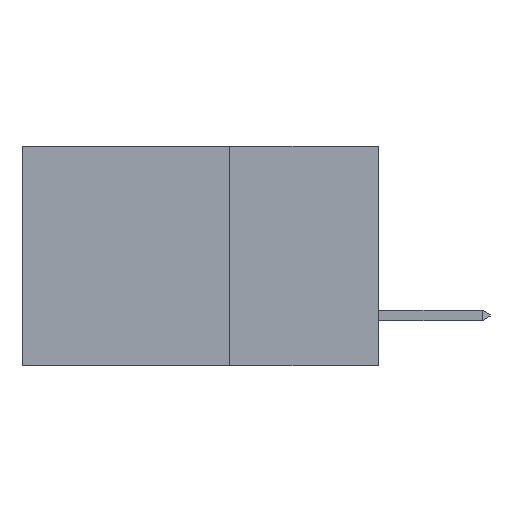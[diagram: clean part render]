
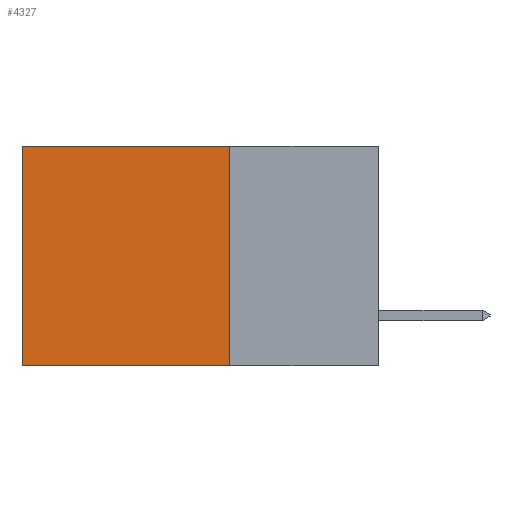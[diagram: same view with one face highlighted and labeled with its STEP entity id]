
A CAD part, left-side view. The second image highlights one B-rep face of the part: STEP entity #4327.
In plain terms, the highlighted planar face has unit normal (-1, 0, 0).
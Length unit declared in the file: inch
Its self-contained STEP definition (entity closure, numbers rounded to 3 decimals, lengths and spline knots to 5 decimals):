
#292 = CARTESIAN_POINT ( 'NONE',  ( 0.298, 0.6, 0. ) ) ;
#398 = ORIENTED_EDGE ( 'NONE', *, *, #7558, .F. ) ;
#803 = CARTESIAN_POINT ( 'NONE',  ( 0.298, 0.25, -0.37 ) ) ;
#1731 = VERTEX_POINT ( 'NONE', #292 ) ;
#1774 = LINE ( 'NONE', #9603, #13063 ) ;
#1909 = PLANE ( 'NONE',  #6850 ) ;
#1918 = DIRECTION ( 'NONE',  ( 0., 1., 0. ) ) ;
#2170 = LINE ( 'NONE', #9643, #13429 ) ;
#2291 = EDGE_CURVE ( 'NONE', #11576, #1731, #2170, .T. ) ;
#2690 = VERTEX_POINT ( 'NONE', #10910 ) ;
#2982 = CARTESIAN_POINT ( 'NONE',  ( 0.298, 0.25, 0. ) ) ;
#4133 = DIRECTION ( 'NONE',  ( 0., 0., -1. ) ) ;
#4327 = ADVANCED_FACE ( 'NONE', ( #7727 ), #1909, .F. ) ;
#5617 = VECTOR ( 'NONE', #13865, 39.37008 ) ;
#6338 = CARTESIAN_POINT ( 'NONE',  ( 0.298, 0.25, 0. ) ) ;
#6403 = ORIENTED_EDGE ( 'NONE', *, *, #2291, .T. ) ;
#6850 = AXIS2_PLACEMENT_3D ( 'NONE', #12520, #6903, #7182 ) ;
#6903 = DIRECTION ( 'NONE',  ( 1., 0., 0. ) ) ;
#7018 = EDGE_LOOP ( 'NONE', ( #10894, #398, #13542, #6403 ) ) ;
#7182 = DIRECTION ( 'NONE',  ( 0., 0., -1. ) ) ;
#7558 = EDGE_CURVE ( 'NONE', #9398, #2690, #1774, .T. ) ;
#7727 = FACE_OUTER_BOUND ( 'NONE', #7018, .T. ) ;
#9398 = VERTEX_POINT ( 'NONE', #803 ) ;
#9548 = CARTESIAN_POINT ( 'NONE',  ( 0.298, 0.6, 0. ) ) ;
#9603 = CARTESIAN_POINT ( 'NONE',  ( 0.298, 0.25, -0.37 ) ) ;
#9643 = CARTESIAN_POINT ( 'NONE',  ( 0.298, 0.25, 0. ) ) ;
#9719 = DIRECTION ( 'NONE',  ( 0., 1., 0. ) ) ;
#10393 = EDGE_CURVE ( 'NONE', #1731, #2690, #12503, .T. ) ;
#10699 = LINE ( 'NONE', #6338, #5617 ) ;
#10894 = ORIENTED_EDGE ( 'NONE', *, *, #10393, .T. ) ;
#10910 = CARTESIAN_POINT ( 'NONE',  ( 0.298, 0.6, -0.37 ) ) ;
#11576 = VERTEX_POINT ( 'NONE', #2982 ) ;
#11857 = VECTOR ( 'NONE', #4133, 39.37008 ) ;
#12503 = LINE ( 'NONE', #9548, #11857 ) ;
#12520 = CARTESIAN_POINT ( 'NONE',  ( 0.298, 0.25, 0. ) ) ;
#13063 = VECTOR ( 'NONE', #1918, 39.37008 ) ;
#13429 = VECTOR ( 'NONE', #9719, 39.37008 ) ;
#13542 = ORIENTED_EDGE ( 'NONE', *, *, #13974, .F. ) ;
#13865 = DIRECTION ( 'NONE',  ( 0., 0., -1. ) ) ;
#13974 = EDGE_CURVE ( 'NONE', #11576, #9398, #10699, .T. ) ;
